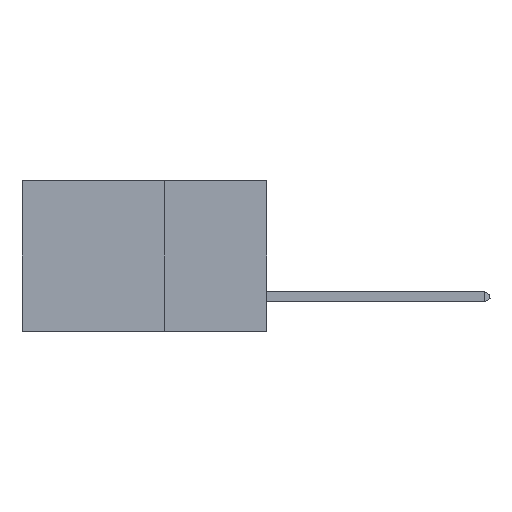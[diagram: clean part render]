
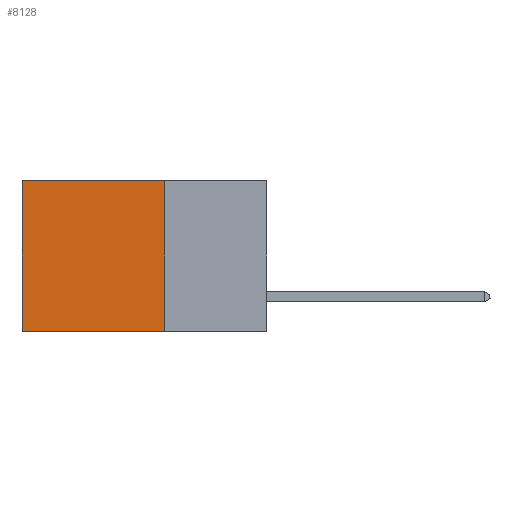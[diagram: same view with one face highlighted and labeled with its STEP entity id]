
A CAD part, left-side view. The second image highlights one B-rep face of the part: STEP entity #8128.
In plain terms, the highlighted planar face has unit normal (-1, 0, 0).
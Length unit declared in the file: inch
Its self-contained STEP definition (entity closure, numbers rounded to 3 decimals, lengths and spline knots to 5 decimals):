
#1076 = VECTOR ( 'NONE', #2945, 39.37008 ) ;
#1328 = EDGE_CURVE ( 'NONE', #13741, #6360, #6080, .T. ) ;
#1381 = DIRECTION ( 'NONE',  ( 0., 0., -1. ) ) ;
#2408 = CARTESIAN_POINT ( 'NONE',  ( 0.2875, 0.25, 0. ) ) ;
#2459 = VERTEX_POINT ( 'NONE', #7621 ) ;
#2460 = PLANE ( 'NONE',  #11788 ) ;
#2721 = EDGE_CURVE ( 'NONE', #6225, #2459, #6399, .T. ) ;
#2945 = DIRECTION ( 'NONE',  ( 0., 1., 0. ) ) ;
#3207 = VECTOR ( 'NONE', #11899, 39.37008 ) ;
#3421 = ORIENTED_EDGE ( 'NONE', *, *, #1328, .T. ) ;
#3495 = CARTESIAN_POINT ( 'NONE',  ( 0.2875, 0.6, 0. ) ) ;
#3505 = VECTOR ( 'NONE', #1381, 39.37008 ) ;
#3592 = DIRECTION ( 'NONE',  ( 0., 0., -1. ) ) ;
#5209 = FACE_OUTER_BOUND ( 'NONE', #11980, .T. ) ;
#5216 = CARTESIAN_POINT ( 'NONE',  ( 0.2875, 0.25, 0. ) ) ;
#5486 = CARTESIAN_POINT ( 'NONE',  ( 0.2875, 0.25, 0. ) ) ;
#6080 = LINE ( 'NONE', #3495, #14397 ) ;
#6128 = LINE ( 'NONE', #5216, #1076 ) ;
#6225 = VERTEX_POINT ( 'NONE', #5486 ) ;
#6360 = VERTEX_POINT ( 'NONE', #12768 ) ;
#6399 = LINE ( 'NONE', #11834, #3505 ) ;
#6411 = ORIENTED_EDGE ( 'NONE', *, *, #2721, .F. ) ;
#7621 = CARTESIAN_POINT ( 'NONE',  ( 0.2875, 0.25, -0.37 ) ) ;
#8128 = ADVANCED_FACE ( 'NONE', ( #5209 ), #2460, .F. ) ;
#8347 = EDGE_CURVE ( 'NONE', #2459, #6360, #13876, .T. ) ;
#10740 = ORIENTED_EDGE ( 'NONE', *, *, #8347, .F. ) ;
#11313 = ORIENTED_EDGE ( 'NONE', *, *, #14498, .T. ) ;
#11753 = DIRECTION ( 'NONE',  ( 1., 0., 0. ) ) ;
#11788 = AXIS2_PLACEMENT_3D ( 'NONE', #2408, #11753, #3592 ) ;
#11834 = CARTESIAN_POINT ( 'NONE',  ( 0.2875, 0.25, 0. ) ) ;
#11899 = DIRECTION ( 'NONE',  ( 0., 1., 0. ) ) ;
#11980 = EDGE_LOOP ( 'NONE', ( #3421, #10740, #6411, #11313 ) ) ;
#12622 = DIRECTION ( 'NONE',  ( 0., 0., -1. ) ) ;
#12768 = CARTESIAN_POINT ( 'NONE',  ( 0.2875, 0.6, -0.37 ) ) ;
#13112 = CARTESIAN_POINT ( 'NONE',  ( 0.2875, 0.25, -0.37 ) ) ;
#13741 = VERTEX_POINT ( 'NONE', #14942 ) ;
#13876 = LINE ( 'NONE', #13112, #3207 ) ;
#14397 = VECTOR ( 'NONE', #12622, 39.37008 ) ;
#14498 = EDGE_CURVE ( 'NONE', #6225, #13741, #6128, .T. ) ;
#14942 = CARTESIAN_POINT ( 'NONE',  ( 0.2875, 0.6, 0. ) ) ;
